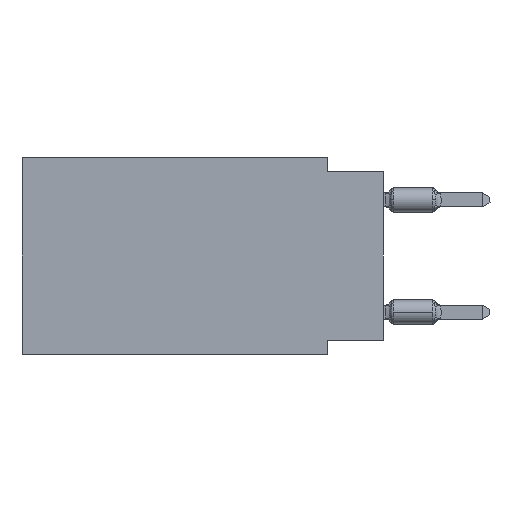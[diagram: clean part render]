
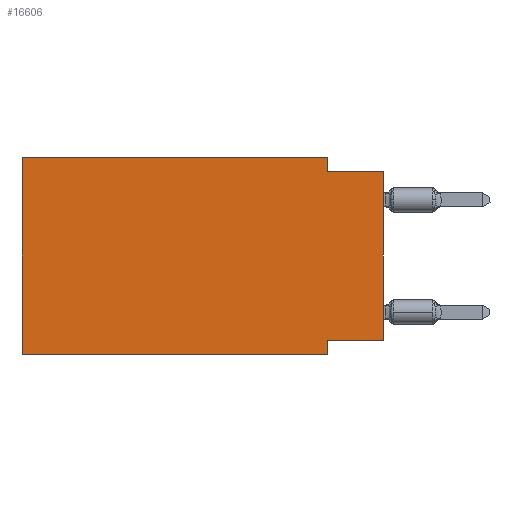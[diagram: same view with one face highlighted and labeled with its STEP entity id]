
A CAD part, left-side view. The second image highlights one B-rep face of the part: STEP entity #16606.
In plain terms, the highlighted planar face has unit normal (-1, 0, 0).
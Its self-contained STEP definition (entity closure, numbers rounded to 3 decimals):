
#182 = ORIENTED_EDGE ( 'NONE', *, *, #437, .F. ) ;
#387 = VECTOR ( 'NONE', #6393, 1000. ) ;
#437 = EDGE_CURVE ( 'NONE', #16294, #3705, #5628, .T. ) ;
#567 = CARTESIAN_POINT ( 'NONE',  ( 0., 0., 0. ) ) ;
#658 = EDGE_CURVE ( 'NONE', #7638, #15500, #2504, .T. ) ;
#842 = VERTEX_POINT ( 'NONE', #3980 ) ;
#1101 = FACE_OUTER_BOUND ( 'NONE', #14614, .T. ) ;
#1988 = LINE ( 'NONE', #11084, #6680 ) ;
#2493 = CARTESIAN_POINT ( 'NONE',  ( 0., 2.54, -8.89 ) ) ;
#2504 = LINE ( 'NONE', #7782, #387 ) ;
#2505 = ORIENTED_EDGE ( 'NONE', *, *, #17027, .F. ) ;
#3200 = VECTOR ( 'NONE', #13227, 1000. ) ;
#3372 = EDGE_CURVE ( 'NONE', #842, #11357, #4870, .T. ) ;
#3705 = VERTEX_POINT ( 'NONE', #9954 ) ;
#3980 = CARTESIAN_POINT ( 'NONE',  ( 0., 2.54, 0. ) ) ;
#4254 = AXIS2_PLACEMENT_3D ( 'NONE', #5166, #5345, #14512 ) ;
#4544 = VECTOR ( 'NONE', #5471, 1000. ) ;
#4870 = LINE ( 'NONE', #8856, #17072 ) ;
#4978 = CARTESIAN_POINT ( 'NONE',  ( 0., 16.383, 0. ) ) ;
#5166 = CARTESIAN_POINT ( 'NONE',  ( 0., 16.383, 0. ) ) ;
#5345 = DIRECTION ( 'NONE',  ( 1., 0., 0. ) ) ;
#5471 = DIRECTION ( 'NONE',  ( 0., 1., 0. ) ) ;
#5628 = LINE ( 'NONE', #8308, #4544 ) ;
#5854 = CARTESIAN_POINT ( 'NONE',  ( 0., 0., -8.255 ) ) ;
#6371 = CARTESIAN_POINT ( 'NONE',  ( 0., 16.383, -8.89 ) ) ;
#6393 = DIRECTION ( 'NONE',  ( 0., -1., 0. ) ) ;
#6680 = VECTOR ( 'NONE', #15063, 1000. ) ;
#6810 = EDGE_CURVE ( 'NONE', #11357, #15199, #1988, .T. ) ;
#7282 = CARTESIAN_POINT ( 'NONE',  ( 0., 2.54, -8.89 ) ) ;
#7638 = VERTEX_POINT ( 'NONE', #6371 ) ;
#7658 = DIRECTION ( 'NONE',  ( 0., -1., 0. ) ) ;
#7782 = CARTESIAN_POINT ( 'NONE',  ( 0., 16.383, -8.89 ) ) ;
#7853 = PLANE ( 'NONE',  #4254 ) ;
#7921 = CARTESIAN_POINT ( 'NONE',  ( 0., 2.54, -0.635 ) ) ;
#8308 = CARTESIAN_POINT ( 'NONE',  ( 0., 0., -8.255 ) ) ;
#8328 = ORIENTED_EDGE ( 'NONE', *, *, #12169, .F. ) ;
#8682 = VECTOR ( 'NONE', #7658, 1000. ) ;
#8715 = EDGE_CURVE ( 'NONE', #16294, #15199, #15191, .T. ) ;
#8811 = ORIENTED_EDGE ( 'NONE', *, *, #6810, .F. ) ;
#8856 = CARTESIAN_POINT ( 'NONE',  ( 0., 2.54, 0. ) ) ;
#8994 = ORIENTED_EDGE ( 'NONE', *, *, #3372, .F. ) ;
#9150 = LINE ( 'NONE', #2493, #3200 ) ;
#9954 = CARTESIAN_POINT ( 'NONE',  ( 0., 2.54, -8.255 ) ) ;
#10240 = ORIENTED_EDGE ( 'NONE', *, *, #12582, .F. ) ;
#10346 = DIRECTION ( 'NONE',  ( 0., 0., 1. ) ) ;
#11084 = CARTESIAN_POINT ( 'NONE',  ( 0., 0., -0.635 ) ) ;
#11357 = VERTEX_POINT ( 'NONE', #7921 ) ;
#11489 = VECTOR ( 'NONE', #16236, 1000. ) ;
#11685 = CARTESIAN_POINT ( 'NONE',  ( 0., 16.383, 0. ) ) ;
#11791 = VECTOR ( 'NONE', #10346, 1000. ) ;
#11996 = ORIENTED_EDGE ( 'NONE', *, *, #658, .T. ) ;
#12169 = EDGE_CURVE ( 'NONE', #3705, #15500, #9150, .T. ) ;
#12582 = EDGE_CURVE ( 'NONE', #7638, #14960, #14138, .T. ) ;
#12840 = DIRECTION ( 'NONE',  ( 0., 0., -1. ) ) ;
#12852 = LINE ( 'NONE', #16997, #8682 ) ;
#13227 = DIRECTION ( 'NONE',  ( 0., 0., -1. ) ) ;
#14138 = LINE ( 'NONE', #4978, #11791 ) ;
#14512 = DIRECTION ( 'NONE',  ( 0., 0., -1. ) ) ;
#14614 = EDGE_LOOP ( 'NONE', ( #15245, #8811, #8994, #2505, #10240, #11996, #8328, #182 ) ) ;
#14960 = VERTEX_POINT ( 'NONE', #11685 ) ;
#15063 = DIRECTION ( 'NONE',  ( 0., -1., 0. ) ) ;
#15191 = LINE ( 'NONE', #567, #11489 ) ;
#15199 = VERTEX_POINT ( 'NONE', #16822 ) ;
#15245 = ORIENTED_EDGE ( 'NONE', *, *, #8715, .T. ) ;
#15500 = VERTEX_POINT ( 'NONE', #7282 ) ;
#16236 = DIRECTION ( 'NONE',  ( 0., 0., 1. ) ) ;
#16294 = VERTEX_POINT ( 'NONE', #5854 ) ;
#16606 = ADVANCED_FACE ( 'NONE', ( #1101 ), #7853, .F. ) ;
#16822 = CARTESIAN_POINT ( 'NONE',  ( 0., 0., -0.635 ) ) ;
#16997 = CARTESIAN_POINT ( 'NONE',  ( 0., 16.383, 0. ) ) ;
#17027 = EDGE_CURVE ( 'NONE', #14960, #842, #12852, .T. ) ;
#17072 = VECTOR ( 'NONE', #12840, 1000. ) ;
